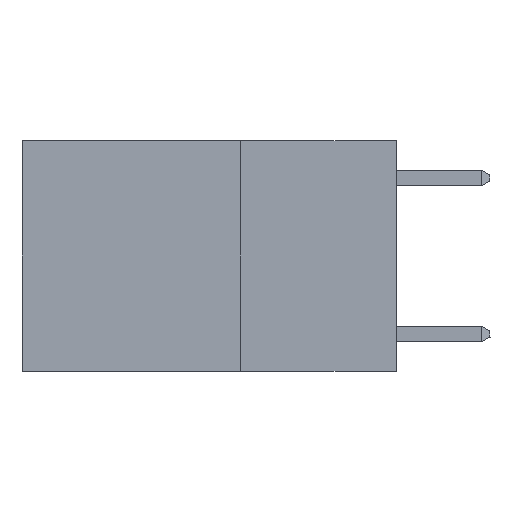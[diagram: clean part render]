
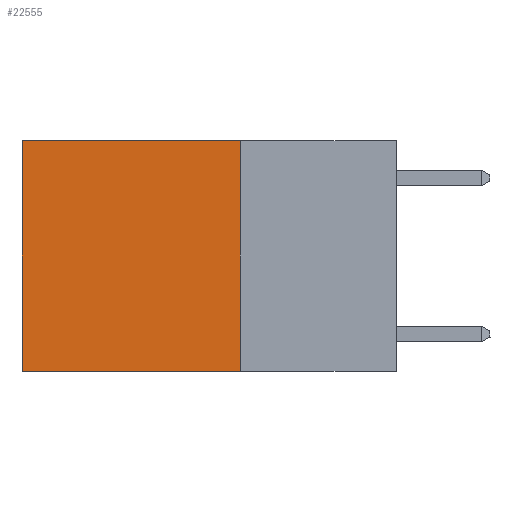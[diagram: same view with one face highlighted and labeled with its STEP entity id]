
A CAD part, left-side view. The second image highlights one B-rep face of the part: STEP entity #22555.
In plain terms, the highlighted planar face has unit normal (-1, 0, 0).
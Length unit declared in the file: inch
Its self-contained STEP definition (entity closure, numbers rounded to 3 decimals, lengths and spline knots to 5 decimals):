
#244 = CARTESIAN_POINT ( 'NONE',  ( 0.2625, 0.6, 0. ) ) ;
#1401 = DIRECTION ( 'NONE',  ( 0., 1., 0. ) ) ;
#1430 = VERTEX_POINT ( 'NONE', #244 ) ;
#2742 = EDGE_LOOP ( 'NONE', ( #6440, #9042, #9066, #9888 ) ) ;
#3040 = EDGE_CURVE ( 'NONE', #16568, #10849, #15311, .T. ) ;
#3403 = EDGE_CURVE ( 'NONE', #10849, #12038, #10927, .T. ) ;
#4641 = CARTESIAN_POINT ( 'NONE',  ( 0.2625, 0.25, 0. ) ) ;
#4805 = DIRECTION ( 'NONE',  ( 0., 0., -1. ) ) ;
#5552 = CARTESIAN_POINT ( 'NONE',  ( 0.2625, 0.25, -0.37 ) ) ;
#5724 = CARTESIAN_POINT ( 'NONE',  ( 0.2625, 0.25, 0. ) ) ;
#5957 = CARTESIAN_POINT ( 'NONE',  ( 0.2625, 0.25, 0. ) ) ;
#6440 = ORIENTED_EDGE ( 'NONE', *, *, #16691, .T. ) ;
#8045 = DIRECTION ( 'NONE',  ( 0., 0., -1. ) ) ;
#8080 = CARTESIAN_POINT ( 'NONE',  ( 0.2625, 0.6, -0.37 ) ) ;
#8757 = DIRECTION ( 'NONE',  ( 0., 0., -1. ) ) ;
#9042 = ORIENTED_EDGE ( 'NONE', *, *, #3403, .F. ) ;
#9066 = ORIENTED_EDGE ( 'NONE', *, *, #3040, .F. ) ;
#9259 = CARTESIAN_POINT ( 'NONE',  ( 0.2625, 0.25, -0.37 ) ) ;
#9374 = EDGE_CURVE ( 'NONE', #16568, #1430, #21408, .T. ) ;
#9888 = ORIENTED_EDGE ( 'NONE', *, *, #9374, .T. ) ;
#9932 = LINE ( 'NONE', #14416, #20011 ) ;
#10849 = VERTEX_POINT ( 'NONE', #5552 ) ;
#10882 = VECTOR ( 'NONE', #18719, 39.37008 ) ;
#10927 = LINE ( 'NONE', #9259, #10882 ) ;
#12038 = VERTEX_POINT ( 'NONE', #8080 ) ;
#14416 = CARTESIAN_POINT ( 'NONE',  ( 0.2625, 0.6, 0. ) ) ;
#15073 = VECTOR ( 'NONE', #4805, 39.37008 ) ;
#15311 = LINE ( 'NONE', #4641, #15073 ) ;
#16154 = CARTESIAN_POINT ( 'NONE',  ( 0.2625, 0.25, 0. ) ) ;
#16568 = VERTEX_POINT ( 'NONE', #16154 ) ;
#16691 = EDGE_CURVE ( 'NONE', #1430, #12038, #9932, .T. ) ;
#18719 = DIRECTION ( 'NONE',  ( 0., 1., 0. ) ) ;
#19408 = DIRECTION ( 'NONE',  ( 1., 0., 0. ) ) ;
#20011 = VECTOR ( 'NONE', #8757, 39.37008 ) ;
#21308 = VECTOR ( 'NONE', #1401, 39.37008 ) ;
#21408 = LINE ( 'NONE', #5724, #21308 ) ;
#22143 = AXIS2_PLACEMENT_3D ( 'NONE', #5957, #19408, #8045 ) ;
#22555 = ADVANCED_FACE ( 'NONE', ( #23612 ), #24535, .F. ) ;
#23612 = FACE_OUTER_BOUND ( 'NONE', #2742, .T. ) ;
#24535 = PLANE ( 'NONE',  #22143 ) ;
